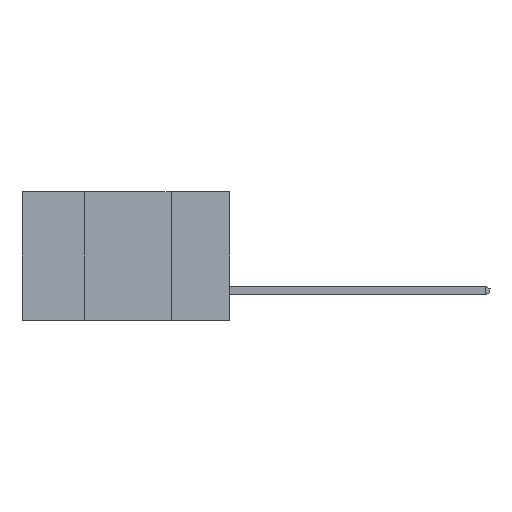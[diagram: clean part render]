
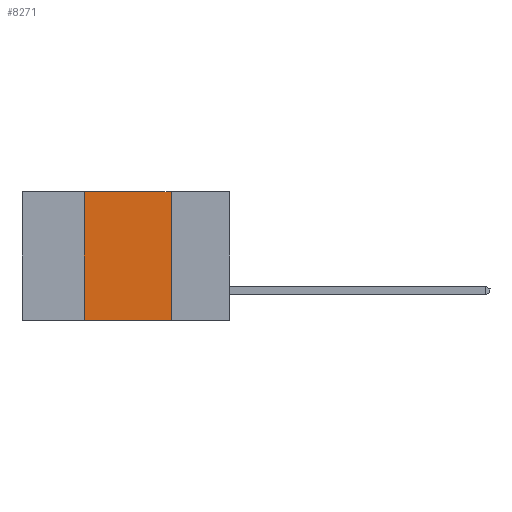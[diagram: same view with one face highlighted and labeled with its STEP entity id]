
A CAD part, left-side view. The second image highlights one B-rep face of the part: STEP entity #8271.
In plain terms, the highlighted planar face has unit normal (-1, 0, 0).
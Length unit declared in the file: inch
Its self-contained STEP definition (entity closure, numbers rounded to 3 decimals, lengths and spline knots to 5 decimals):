
#539 = VECTOR ( 'NONE', #10821, 39.37008 ) ;
#594 = ORIENTED_EDGE ( 'NONE', *, *, #7752, .F. ) ;
#670 = CARTESIAN_POINT ( 'NONE',  ( 0., 0.17, 0. ) ) ;
#894 = CARTESIAN_POINT ( 'NONE',  ( 0., 0.6, 0. ) ) ;
#1138 = ORIENTED_EDGE ( 'NONE', *, *, #6642, .T. ) ;
#1143 = CARTESIAN_POINT ( 'NONE',  ( 0., 0.42, -0.37 ) ) ;
#1309 = DIRECTION ( 'NONE',  ( 0., 0., 1. ) ) ;
#1786 = DIRECTION ( 'NONE',  ( 0., 0., -1. ) ) ;
#2237 = LINE ( 'NONE', #7360, #4530 ) ;
#2284 = VERTEX_POINT ( 'NONE', #670 ) ;
#2919 = CARTESIAN_POINT ( 'NONE',  ( 0., 0.17, 0. ) ) ;
#3169 = CARTESIAN_POINT ( 'NONE',  ( 0., 0.6, -0.37 ) ) ;
#3207 = LINE ( 'NONE', #8323, #539 ) ;
#3710 = VECTOR ( 'NONE', #10457, 39.37008 ) ;
#4530 = VECTOR ( 'NONE', #1309, 39.37008 ) ;
#4837 = LINE ( 'NONE', #3169, #8996 ) ;
#5453 = CARTESIAN_POINT ( 'NONE',  ( 0., 0.17, -0.37 ) ) ;
#5520 = VERTEX_POINT ( 'NONE', #1143 ) ;
#6005 = FACE_OUTER_BOUND ( 'NONE', #7466, .T. ) ;
#6012 = LINE ( 'NONE', #2919, #3710 ) ;
#6517 = AXIS2_PLACEMENT_3D ( 'NONE', #894, #6961, #1786 ) ;
#6618 = VERTEX_POINT ( 'NONE', #10653 ) ;
#6642 = EDGE_CURVE ( 'NONE', #5520, #6984, #4837, .T. ) ;
#6961 = DIRECTION ( 'NONE',  ( 1., 0., 0. ) ) ;
#6984 = VERTEX_POINT ( 'NONE', #5453 ) ;
#7189 = EDGE_CURVE ( 'NONE', #5520, #6618, #2237, .T. ) ;
#7342 = EDGE_CURVE ( 'NONE', #6618, #2284, #3207, .T. ) ;
#7360 = CARTESIAN_POINT ( 'NONE',  ( 0., 0.42, 0. ) ) ;
#7415 = DIRECTION ( 'NONE',  ( 0., -1., 0. ) ) ;
#7466 = EDGE_LOOP ( 'NONE', ( #594, #7521, #9946, #1138 ) ) ;
#7521 = ORIENTED_EDGE ( 'NONE', *, *, #7342, .F. ) ;
#7752 = EDGE_CURVE ( 'NONE', #2284, #6984, #6012, .T. ) ;
#8271 = ADVANCED_FACE ( 'NONE', ( #6005 ), #10246, .F. ) ;
#8323 = CARTESIAN_POINT ( 'NONE',  ( 0., 0.6, 0. ) ) ;
#8996 = VECTOR ( 'NONE', #7415, 39.37008 ) ;
#9946 = ORIENTED_EDGE ( 'NONE', *, *, #7189, .F. ) ;
#10246 = PLANE ( 'NONE',  #6517 ) ;
#10457 = DIRECTION ( 'NONE',  ( 0., 0., -1. ) ) ;
#10653 = CARTESIAN_POINT ( 'NONE',  ( 0., 0.42, 0. ) ) ;
#10821 = DIRECTION ( 'NONE',  ( 0., -1., 0. ) ) ;
